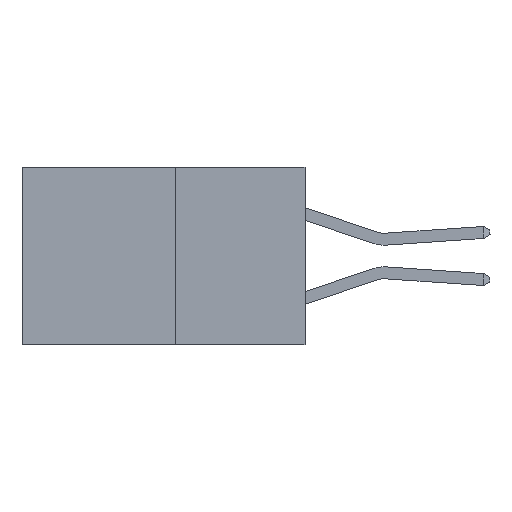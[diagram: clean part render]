
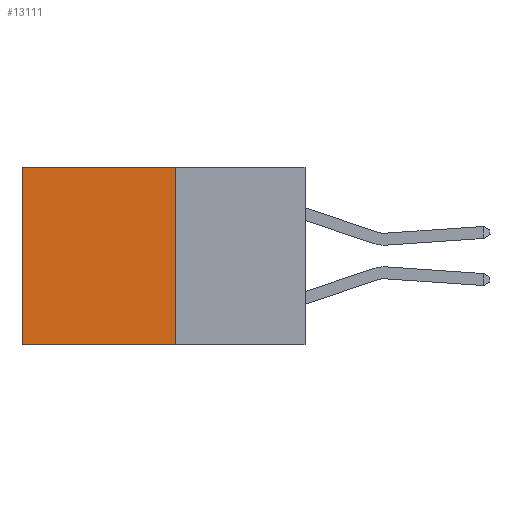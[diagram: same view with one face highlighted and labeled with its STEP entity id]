
A CAD part, left-side view. The second image highlights one B-rep face of the part: STEP entity #13111.
In plain terms, the highlighted planar face has unit normal (-1, 0, 0).
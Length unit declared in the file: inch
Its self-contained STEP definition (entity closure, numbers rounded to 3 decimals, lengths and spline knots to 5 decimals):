
#552 = CARTESIAN_POINT ( 'NONE',  ( 0.277, 0.59, 0. ) ) ;
#554 = DIRECTION ( 'NONE',  ( 1., 0., 0. ) ) ;
#755 = DIRECTION ( 'NONE',  ( 0., 1., 0. ) ) ;
#1360 = CARTESIAN_POINT ( 'NONE',  ( 0.277, 0.59, -0.37 ) ) ;
#1374 = EDGE_CURVE ( 'NONE', #10235, #4397, #13042, .T. ) ;
#1986 = CARTESIAN_POINT ( 'NONE',  ( 0.277, 0.27, 0. ) ) ;
#2636 = ORIENTED_EDGE ( 'NONE', *, *, #1374, .T. ) ;
#2783 = FACE_OUTER_BOUND ( 'NONE', #9078, .T. ) ;
#4193 = LINE ( 'NONE', #5430, #6593 ) ;
#4397 = VERTEX_POINT ( 'NONE', #552 ) ;
#4958 = EDGE_CURVE ( 'NONE', #4397, #12914, #4193, .T. ) ;
#5430 = CARTESIAN_POINT ( 'NONE',  ( 0.277, 0.59, -0.37 ) ) ;
#5496 = CARTESIAN_POINT ( 'NONE',  ( 0.277, 0.27, 0. ) ) ;
#5611 = DIRECTION ( 'NONE',  ( 0., 1., 0. ) ) ;
#5625 = CARTESIAN_POINT ( 'NONE',  ( 0.277, 0.27, -0.37 ) ) ;
#5797 = VECTOR ( 'NONE', #7303, 39.37008 ) ;
#6215 = CARTESIAN_POINT ( 'NONE',  ( 0.277, 0.27, -0.37 ) ) ;
#6565 = LINE ( 'NONE', #5625, #12082 ) ;
#6593 = VECTOR ( 'NONE', #13015, 39.37008 ) ;
#6904 = ORIENTED_EDGE ( 'NONE', *, *, #11491, .F. ) ;
#7190 = EDGE_CURVE ( 'NONE', #8588, #12914, #6565, .T. ) ;
#7303 = DIRECTION ( 'NONE',  ( 0., 0., -1. ) ) ;
#7410 = ORIENTED_EDGE ( 'NONE', *, *, #7190, .F. ) ;
#7831 = VECTOR ( 'NONE', #755, 39.37008 ) ;
#8000 = DIRECTION ( 'NONE',  ( 0., 0., -1. ) ) ;
#8588 = VERTEX_POINT ( 'NONE', #6215 ) ;
#8618 = LINE ( 'NONE', #9390, #5797 ) ;
#9078 = EDGE_LOOP ( 'NONE', ( #9867, #7410, #6904, #2636 ) ) ;
#9390 = CARTESIAN_POINT ( 'NONE',  ( 0.277, 0.27, -0.37 ) ) ;
#9867 = ORIENTED_EDGE ( 'NONE', *, *, #4958, .T. ) ;
#10235 = VERTEX_POINT ( 'NONE', #5496 ) ;
#11491 = EDGE_CURVE ( 'NONE', #10235, #8588, #8618, .T. ) ;
#11745 = AXIS2_PLACEMENT_3D ( 'NONE', #13190, #554, #8000 ) ;
#12082 = VECTOR ( 'NONE', #5611, 39.37008 ) ;
#12104 = PLANE ( 'NONE',  #11745 ) ;
#12914 = VERTEX_POINT ( 'NONE', #1360 ) ;
#13015 = DIRECTION ( 'NONE',  ( 0., 0., -1. ) ) ;
#13042 = LINE ( 'NONE', #1986, #7831 ) ;
#13111 = ADVANCED_FACE ( 'NONE', ( #2783 ), #12104, .F. ) ;
#13190 = CARTESIAN_POINT ( 'NONE',  ( 0.277, 0.27, -0.37 ) ) ;
